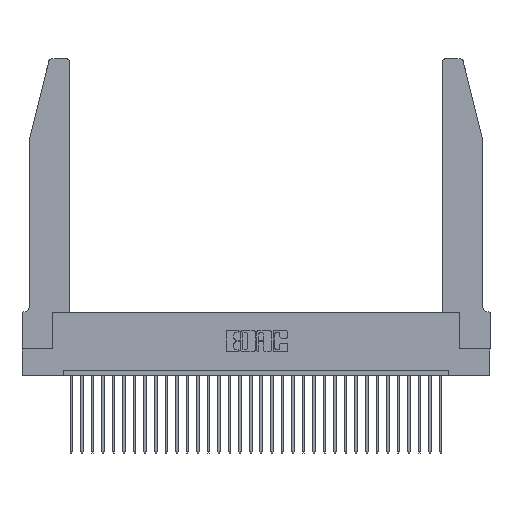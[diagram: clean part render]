
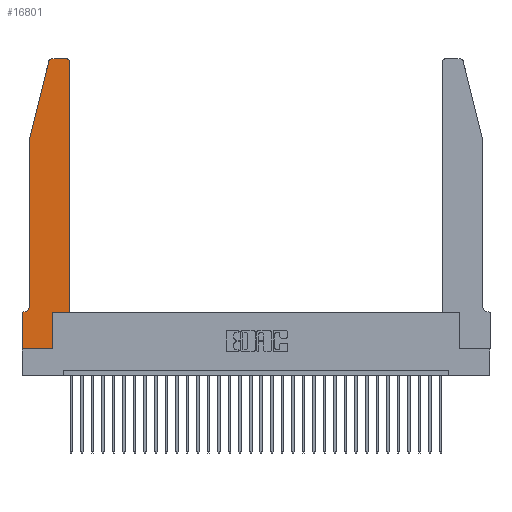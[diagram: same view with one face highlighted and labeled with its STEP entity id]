
A CAD part, top view. The second image highlights one B-rep face of the part: STEP entity #16801.
In plain terms, the highlighted planar face has unit normal (0, 0, 1).
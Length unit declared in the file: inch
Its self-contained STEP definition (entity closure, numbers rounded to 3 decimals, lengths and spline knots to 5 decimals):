
#322 = VERTEX_POINT ( 'NONE', #23088 ) ;
#465 = CARTESIAN_POINT ( 'NONE',  ( 0.0755, 0.35, 0.37 ) ) ;
#736 = VERTEX_POINT ( 'NONE', #5548 ) ;
#950 = ORIENTED_EDGE ( 'NONE', *, *, #22772, .T. ) ;
#1918 = CIRCLE ( 'NONE', #28294, 0.03 ) ;
#2145 = LINE ( 'NONE', #3150, #6124 ) ;
#2224 = DIRECTION ( 'NONE',  ( 1., 0., 0. ) ) ;
#3150 = CARTESIAN_POINT ( 'NONE',  ( 0., 0., 0.37 ) ) ;
#3166 = ORIENTED_EDGE ( 'NONE', *, *, #32145, .T. ) ;
#3699 = ORIENTED_EDGE ( 'NONE', *, *, #24008, .T. ) ;
#4083 = VECTOR ( 'NONE', #13228, 39.37008 ) ;
#4180 = VERTEX_POINT ( 'NONE', #5298 ) ;
#4872 = DIRECTION ( 'NONE',  ( 0., 0., 1. ) ) ;
#5088 = EDGE_CURVE ( 'NONE', #24800, #16388, #17921, .T. ) ;
#5115 = LINE ( 'NONE', #11087, #17849 ) ;
#5169 = CIRCLE ( 'NONE', #11260, 0.03 ) ;
#5298 = CARTESIAN_POINT ( 'NONE',  ( 0., 0., 0.37 ) ) ;
#5548 = CARTESIAN_POINT ( 'NONE',  ( 0.25487, 2.72718, 0.37 ) ) ;
#5553 = VERTEX_POINT ( 'NONE', #17076 ) ;
#5573 = VERTEX_POINT ( 'NONE', #22201 ) ;
#5831 = ORIENTED_EDGE ( 'NONE', *, *, #31716, .T. ) ;
#5857 = DIRECTION ( 'NONE',  ( 1., 0., 0. ) ) ;
#5896 = CARTESIAN_POINT ( 'NONE',  ( 0.2865, 0.35, 0.37 ) ) ;
#6124 = VECTOR ( 'NONE', #5857, 39.37008 ) ;
#6168 = ORIENTED_EDGE ( 'NONE', *, *, #8011, .T. ) ;
#6365 = DIRECTION ( 'NONE',  ( 0., 1., 0. ) ) ;
#6470 = DIRECTION ( 'NONE',  ( -0.239, -0.971, 0. ) ) ;
#6993 = VECTOR ( 'NONE', #13580, 39.37008 ) ;
#7587 = ORIENTED_EDGE ( 'NONE', *, *, #25173, .T. ) ;
#8011 = EDGE_CURVE ( 'NONE', #18457, #24800, #23370, .T. ) ;
#8126 = VECTOR ( 'NONE', #6470, 39.37008 ) ;
#8200 = CARTESIAN_POINT ( 'NONE',  ( 0.2865, 0.35, 0.37 ) ) ;
#8246 = ORIENTED_EDGE ( 'NONE', *, *, #9021, .T. ) ;
#9021 = EDGE_CURVE ( 'NONE', #16388, #17872, #5169, .T. ) ;
#9402 = CARTESIAN_POINT ( 'NONE',  ( 0.4505, 0.35, 0.37 ) ) ;
#9495 = DIRECTION ( 'NONE',  ( 0., -1., 0. ) ) ;
#9532 = CARTESIAN_POINT ( 'NONE',  ( 0.4205, 2.75, 0.37 ) ) ;
#9631 = CARTESIAN_POINT ( 'NONE',  ( 0.2605, 2.75, 0.37 ) ) ;
#9837 = CARTESIAN_POINT ( 'NONE',  ( 0.0755, 0.42, 0.37 ) ) ;
#10333 = AXIS2_PLACEMENT_3D ( 'NONE', #21630, #31751, #21738 ) ;
#10814 = VECTOR ( 'NONE', #2224, 39.37008 ) ;
#11087 = CARTESIAN_POINT ( 'NONE',  ( 0., 0., 0.37 ) ) ;
#11260 = AXIS2_PLACEMENT_3D ( 'NONE', #22146, #31942, #27285 ) ;
#11488 = VERTEX_POINT ( 'NONE', #14951 ) ;
#11604 = CARTESIAN_POINT ( 'NONE',  ( 0.4505, 0.35, 0.37 ) ) ;
#11657 = EDGE_LOOP ( 'NONE', ( #29720, #950, #5831, #27293, #12858, #3699, #3166, #31209, #7587, #6168, #16214, #8246 ) ) ;
#12123 = CARTESIAN_POINT ( 'NONE',  ( 0.4505, 0.35, 0.37 ) ) ;
#12295 = DIRECTION ( 'NONE',  ( -1., 0., 0. ) ) ;
#12476 = LINE ( 'NONE', #8200, #4083 ) ;
#12858 = ORIENTED_EDGE ( 'NONE', *, *, #20101, .T. ) ;
#13047 = VERTEX_POINT ( 'NONE', #29904 ) ;
#13228 = DIRECTION ( 'NONE',  ( 0., 1., 0. ) ) ;
#13580 = DIRECTION ( 'NONE',  ( -1., 0., 0. ) ) ;
#13692 = EDGE_CURVE ( 'NONE', #4180, #11488, #2145, .T. ) ;
#14425 = VECTOR ( 'NONE', #6365, 39.37008 ) ;
#14951 = CARTESIAN_POINT ( 'NONE',  ( 0.2865, 0., 0.37 ) ) ;
#15194 = EDGE_CURVE ( 'NONE', #13047, #24901, #31636, .T. ) ;
#16180 = LINE ( 'NONE', #9631, #18925 ) ;
#16214 = ORIENTED_EDGE ( 'NONE', *, *, #5088, .T. ) ;
#16388 = VERTEX_POINT ( 'NONE', #19535 ) ;
#16801 = ADVANCED_FACE ( 'NONE', ( #31977 ), #31644, .T. ) ;
#17076 = CARTESIAN_POINT ( 'NONE',  ( 0., 0.35, 0.37 ) ) ;
#17516 = CARTESIAN_POINT ( 'NONE',  ( 0.284, 2.72, 0.37 ) ) ;
#17849 = VECTOR ( 'NONE', #28311, 39.37008 ) ;
#17872 = VERTEX_POINT ( 'NONE', #9532 ) ;
#17898 = EDGE_CURVE ( 'NONE', #17872, #322, #16180, .T. ) ;
#17921 = LINE ( 'NONE', #11604, #14425 ) ;
#18027 = LINE ( 'NONE', #26823, #8126 ) ;
#18457 = VERTEX_POINT ( 'NONE', #5896 ) ;
#18561 = DIRECTION ( 'NONE',  ( 0., 0., -1. ) ) ;
#18925 = VECTOR ( 'NONE', #12295, 39.37008 ) ;
#19019 = CARTESIAN_POINT ( 'NONE',  ( 0.0055, 0.42, 0.37 ) ) ;
#19535 = CARTESIAN_POINT ( 'NONE',  ( 0.4505, 2.72, 0.37 ) ) ;
#20101 = EDGE_CURVE ( 'NONE', #24901, #5573, #23691, .T. ) ;
#21372 = DIRECTION ( 'NONE',  ( -1., 0., 0. ) ) ;
#21630 = CARTESIAN_POINT ( 'NONE',  ( 0., 0.35, 0.37 ) ) ;
#21738 = DIRECTION ( 'NONE',  ( 1., 0., 0. ) ) ;
#22146 = CARTESIAN_POINT ( 'NONE',  ( 0.4205, 2.72, 0.37 ) ) ;
#22201 = CARTESIAN_POINT ( 'NONE',  ( 0.0055, 0.35, 0.37 ) ) ;
#22336 = LINE ( 'NONE', #465, #6993 ) ;
#22519 = DIRECTION ( 'NONE',  ( 1., 0., 0. ) ) ;
#22772 = EDGE_CURVE ( 'NONE', #322, #736, #1918, .T. ) ;
#23088 = CARTESIAN_POINT ( 'NONE',  ( 0.284, 2.75, 0.37 ) ) ;
#23370 = LINE ( 'NONE', #12123, #10814 ) ;
#23691 = CIRCLE ( 'NONE', #26776, 0.07 ) ;
#24008 = EDGE_CURVE ( 'NONE', #5573, #5553, #22336, .T. ) ;
#24727 = CARTESIAN_POINT ( 'NONE',  ( 0.0755, 2., 0.37 ) ) ;
#24800 = VERTEX_POINT ( 'NONE', #9402 ) ;
#24901 = VERTEX_POINT ( 'NONE', #9837 ) ;
#25173 = EDGE_CURVE ( 'NONE', #11488, #18457, #12476, .T. ) ;
#26776 = AXIS2_PLACEMENT_3D ( 'NONE', #19019, #18561, #21372 ) ;
#26823 = CARTESIAN_POINT ( 'NONE',  ( 0.0755, 2., 0.37 ) ) ;
#27285 = DIRECTION ( 'NONE',  ( 1., 0., 0. ) ) ;
#27293 = ORIENTED_EDGE ( 'NONE', *, *, #15194, .T. ) ;
#28294 = AXIS2_PLACEMENT_3D ( 'NONE', #17516, #4872, #22519 ) ;
#28311 = DIRECTION ( 'NONE',  ( 0., -1., 0. ) ) ;
#29720 = ORIENTED_EDGE ( 'NONE', *, *, #17898, .T. ) ;
#29904 = CARTESIAN_POINT ( 'NONE',  ( 0.0755, 2., 0.37 ) ) ;
#31209 = ORIENTED_EDGE ( 'NONE', *, *, #13692, .T. ) ;
#31636 = LINE ( 'NONE', #24727, #32461 ) ;
#31644 = PLANE ( 'NONE',  #10333 ) ;
#31716 = EDGE_CURVE ( 'NONE', #736, #13047, #18027, .T. ) ;
#31751 = DIRECTION ( 'NONE',  ( 0., 0., 1. ) ) ;
#31942 = DIRECTION ( 'NONE',  ( 0., 0., 1. ) ) ;
#31977 = FACE_OUTER_BOUND ( 'NONE', #11657, .T. ) ;
#32145 = EDGE_CURVE ( 'NONE', #5553, #4180, #5115, .T. ) ;
#32461 = VECTOR ( 'NONE', #9495, 39.37008 ) ;
